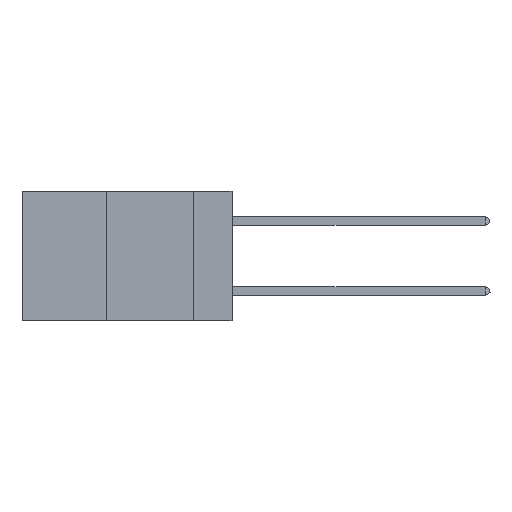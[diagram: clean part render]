
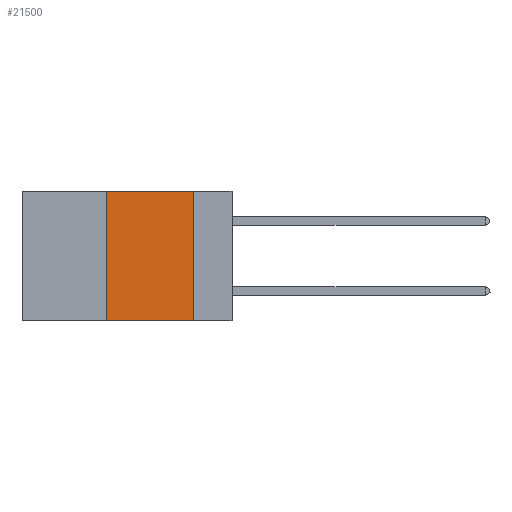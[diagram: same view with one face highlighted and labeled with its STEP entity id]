
A CAD part, left-side view. The second image highlights one B-rep face of the part: STEP entity #21500.
In plain terms, the highlighted planar face has unit normal (-1, 0, 0).
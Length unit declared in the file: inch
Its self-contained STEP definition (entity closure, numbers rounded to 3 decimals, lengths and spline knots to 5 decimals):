
#213 = CARTESIAN_POINT ( 'NONE',  ( 0., 0.6, -0.37 ) ) ;
#1277 = DIRECTION ( 'NONE',  ( 1., 0., 0. ) ) ;
#1319 = LINE ( 'NONE', #21952, #20583 ) ;
#1661 = CARTESIAN_POINT ( 'NONE',  ( 0., 0.11, 0. ) ) ;
#3161 = PLANE ( 'NONE',  #12829 ) ;
#3234 = ORIENTED_EDGE ( 'NONE', *, *, #22013, .F. ) ;
#4919 = DIRECTION ( 'NONE',  ( 0., 0., -1. ) ) ;
#5916 = CARTESIAN_POINT ( 'NONE',  ( 0., 0.11, 0. ) ) ;
#8953 = FACE_OUTER_BOUND ( 'NONE', #16922, .T. ) ;
#9349 = VERTEX_POINT ( 'NONE', #9743 ) ;
#9743 = CARTESIAN_POINT ( 'NONE',  ( 0., 0.36, -0.37 ) ) ;
#9805 = VERTEX_POINT ( 'NONE', #16208 ) ;
#9998 = VECTOR ( 'NONE', #12071, 39.37008 ) ;
#10665 = ORIENTED_EDGE ( 'NONE', *, *, #16346, .T. ) ;
#10793 = ORIENTED_EDGE ( 'NONE', *, *, #11875, .F. ) ;
#11875 = EDGE_CURVE ( 'NONE', #17789, #12866, #14448, .T. ) ;
#12071 = DIRECTION ( 'NONE',  ( 0., 0., -1. ) ) ;
#12377 = DIRECTION ( 'NONE',  ( 0., -1., 0. ) ) ;
#12829 = AXIS2_PLACEMENT_3D ( 'NONE', #15258, #1277, #4919 ) ;
#12866 = VERTEX_POINT ( 'NONE', #5916 ) ;
#14448 = LINE ( 'NONE', #18641, #21815 ) ;
#14482 = EDGE_CURVE ( 'NONE', #12866, #9805, #21401, .T. ) ;
#14811 = VECTOR ( 'NONE', #12377, 39.37008 ) ;
#15258 = CARTESIAN_POINT ( 'NONE',  ( 0., 0.6, 0. ) ) ;
#16208 = CARTESIAN_POINT ( 'NONE',  ( 0., 0.11, -0.37 ) ) ;
#16346 = EDGE_CURVE ( 'NONE', #9349, #9805, #19989, .T. ) ;
#16922 = EDGE_LOOP ( 'NONE', ( #21030, #10793, #3234, #10665 ) ) ;
#17037 = CARTESIAN_POINT ( 'NONE',  ( 0., 0.36, 0. ) ) ;
#17789 = VERTEX_POINT ( 'NONE', #17037 ) ;
#18641 = CARTESIAN_POINT ( 'NONE',  ( 0., 0.6, 0. ) ) ;
#18872 = DIRECTION ( 'NONE',  ( 0., -1., 0. ) ) ;
#19989 = LINE ( 'NONE', #213, #14811 ) ;
#20583 = VECTOR ( 'NONE', #21402, 39.37008 ) ;
#21030 = ORIENTED_EDGE ( 'NONE', *, *, #14482, .F. ) ;
#21401 = LINE ( 'NONE', #1661, #9998 ) ;
#21402 = DIRECTION ( 'NONE',  ( 0., 0., 1. ) ) ;
#21500 = ADVANCED_FACE ( 'NONE', ( #8953 ), #3161, .F. ) ;
#21815 = VECTOR ( 'NONE', #18872, 39.37008 ) ;
#21952 = CARTESIAN_POINT ( 'NONE',  ( 0., 0.36, 0. ) ) ;
#22013 = EDGE_CURVE ( 'NONE', #9349, #17789, #1319, .T. ) ;
